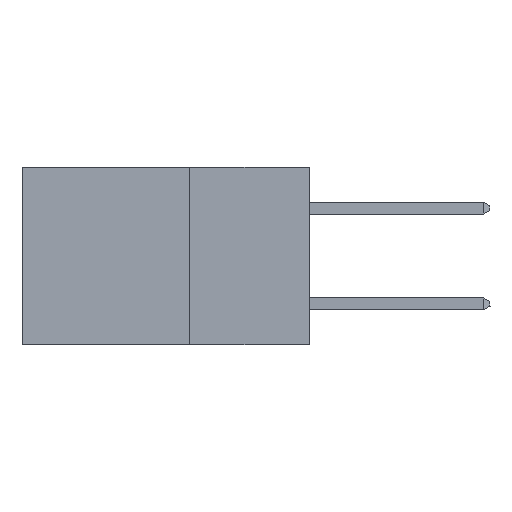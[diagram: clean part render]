
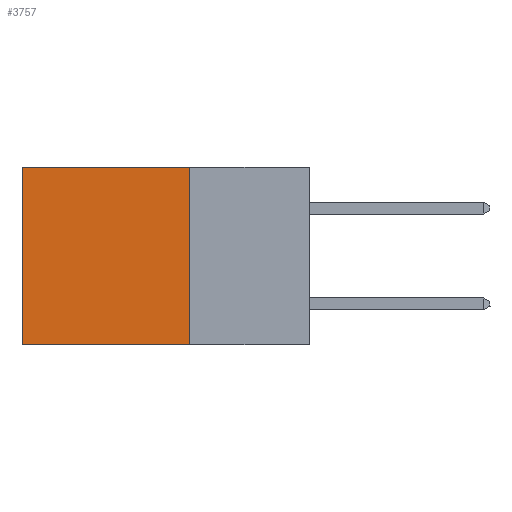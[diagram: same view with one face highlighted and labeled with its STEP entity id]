
A CAD part, left-side view. The second image highlights one B-rep face of the part: STEP entity #3757.
In plain terms, the highlighted planar face has unit normal (-1, 0, 0).
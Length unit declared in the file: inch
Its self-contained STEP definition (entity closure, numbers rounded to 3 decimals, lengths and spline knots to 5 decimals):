
#1221 = LINE ( 'NONE', #16560, #20745 ) ;
#1773 = CARTESIAN_POINT ( 'NONE',  ( 0.2875, 0.25, 0. ) ) ;
#2442 = FACE_OUTER_BOUND ( 'NONE', #5076, .T. ) ;
#3010 = DIRECTION ( 'NONE',  ( 0., 1., 0. ) ) ;
#3757 = ADVANCED_FACE ( 'NONE', ( #2442 ), #30423, .F. ) ;
#5076 = EDGE_LOOP ( 'NONE', ( #18298, #27057, #11441, #24313 ) ) ;
#5656 = VECTOR ( 'NONE', #3010, 39.37008 ) ;
#5860 = VERTEX_POINT ( 'NONE', #1773 ) ;
#6770 = CARTESIAN_POINT ( 'NONE',  ( 0.2875, 0.25, 0. ) ) ;
#7238 = VERTEX_POINT ( 'NONE', #16363 ) ;
#7751 = CARTESIAN_POINT ( 'NONE',  ( 0.2875, 0.6, -0.37 ) ) ;
#8913 = EDGE_CURVE ( 'NONE', #5860, #7238, #20959, .T. ) ;
#10021 = VECTOR ( 'NONE', #12435, 39.37008 ) ;
#10479 = DIRECTION ( 'NONE',  ( 0., 0., -1. ) ) ;
#10558 = LINE ( 'NONE', #33597, #5656 ) ;
#11031 = VERTEX_POINT ( 'NONE', #7751 ) ;
#11441 = ORIENTED_EDGE ( 'NONE', *, *, #8913, .F. ) ;
#12435 = DIRECTION ( 'NONE',  ( 0., 1., 0. ) ) ;
#14500 = EDGE_CURVE ( 'NONE', #7238, #11031, #17060, .T. ) ;
#16363 = CARTESIAN_POINT ( 'NONE',  ( 0.2875, 0.25, -0.37 ) ) ;
#16560 = CARTESIAN_POINT ( 'NONE',  ( 0.2875, 0.6, 0. ) ) ;
#17060 = LINE ( 'NONE', #32620, #10021 ) ;
#18298 = ORIENTED_EDGE ( 'NONE', *, *, #26969, .T. ) ;
#19654 = DIRECTION ( 'NONE',  ( 0., 0., -1. ) ) ;
#20745 = VECTOR ( 'NONE', #19654, 39.37008 ) ;
#20959 = LINE ( 'NONE', #6770, #35239 ) ;
#21758 = CARTESIAN_POINT ( 'NONE',  ( 0.2875, 0.25, 0. ) ) ;
#22003 = DIRECTION ( 'NONE',  ( 1., 0., 0. ) ) ;
#24313 = ORIENTED_EDGE ( 'NONE', *, *, #35130, .T. ) ;
#26969 = EDGE_CURVE ( 'NONE', #27098, #11031, #1221, .T. ) ;
#27057 = ORIENTED_EDGE ( 'NONE', *, *, #14500, .F. ) ;
#27098 = VERTEX_POINT ( 'NONE', #28449 ) ;
#27199 = AXIS2_PLACEMENT_3D ( 'NONE', #21758, #22003, #10479 ) ;
#28449 = CARTESIAN_POINT ( 'NONE',  ( 0.2875, 0.6, 0. ) ) ;
#30423 = PLANE ( 'NONE',  #27199 ) ;
#32061 = DIRECTION ( 'NONE',  ( 0., 0., -1. ) ) ;
#32620 = CARTESIAN_POINT ( 'NONE',  ( 0.2875, 0.25, -0.37 ) ) ;
#33597 = CARTESIAN_POINT ( 'NONE',  ( 0.2875, 0.25, 0. ) ) ;
#35130 = EDGE_CURVE ( 'NONE', #5860, #27098, #10558, .T. ) ;
#35239 = VECTOR ( 'NONE', #32061, 39.37008 ) ;
